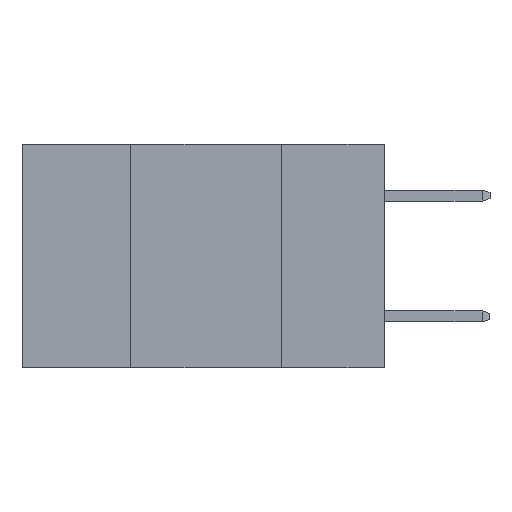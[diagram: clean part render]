
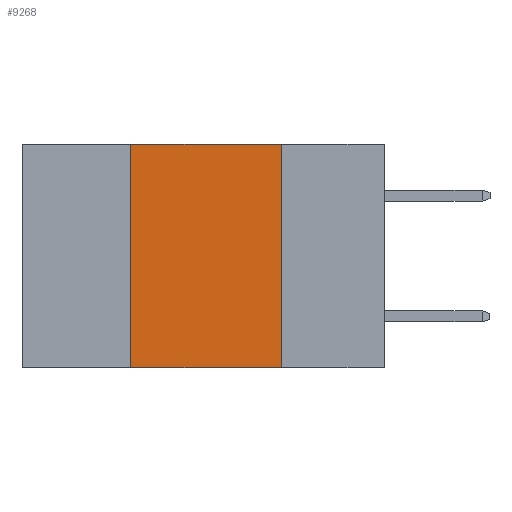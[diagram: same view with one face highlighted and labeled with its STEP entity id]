
A CAD part, left-side view. The second image highlights one B-rep face of the part: STEP entity #9268.
In plain terms, the highlighted planar face has unit normal (-1, 0, 0).
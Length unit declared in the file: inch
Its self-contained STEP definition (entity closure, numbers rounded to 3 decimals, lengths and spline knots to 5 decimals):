
#30 = EDGE_LOOP ( 'NONE', ( #9374, #10619, #9233, #5030 ) ) ;
#102 = VERTEX_POINT ( 'NONE', #7664 ) ;
#133 = CARTESIAN_POINT ( 'NONE',  ( 0., 0.42, 0. ) ) ;
#432 = CARTESIAN_POINT ( 'NONE',  ( 0., 0.6, -0.37 ) ) ;
#594 = CARTESIAN_POINT ( 'NONE',  ( 0., 0.42, 0. ) ) ;
#979 = EDGE_CURVE ( 'NONE', #102, #9115, #9741, .T. ) ;
#1003 = DIRECTION ( 'NONE',  ( 0., 0., 1. ) ) ;
#1593 = DIRECTION ( 'NONE',  ( 0., -1., 0. ) ) ;
#1744 = VECTOR ( 'NONE', #5534, 39.37008 ) ;
#2092 = AXIS2_PLACEMENT_3D ( 'NONE', #9020, #3743, #9863 ) ;
#2441 = LINE ( 'NONE', #133, #8982 ) ;
#2707 = VECTOR ( 'NONE', #3773, 39.37008 ) ;
#2812 = PLANE ( 'NONE',  #2092 ) ;
#3152 = VERTEX_POINT ( 'NONE', #594 ) ;
#3743 = DIRECTION ( 'NONE',  ( 1., 0., 0. ) ) ;
#3773 = DIRECTION ( 'NONE',  ( 0., -1., 0. ) ) ;
#3860 = LINE ( 'NONE', #4650, #1744 ) ;
#4650 = CARTESIAN_POINT ( 'NONE',  ( 0., 0.17, 0. ) ) ;
#5030 = ORIENTED_EDGE ( 'NONE', *, *, #979, .T. ) ;
#5378 = LINE ( 'NONE', #6963, #7765 ) ;
#5534 = DIRECTION ( 'NONE',  ( 0., 0., -1. ) ) ;
#5573 = CARTESIAN_POINT ( 'NONE',  ( 0., 0.17, 0. ) ) ;
#5905 = EDGE_CURVE ( 'NONE', #3152, #10644, #5378, .T. ) ;
#6963 = CARTESIAN_POINT ( 'NONE',  ( 0., 0.6, 0. ) ) ;
#7664 = CARTESIAN_POINT ( 'NONE',  ( 0., 0.42, -0.37 ) ) ;
#7765 = VECTOR ( 'NONE', #1593, 39.37008 ) ;
#8982 = VECTOR ( 'NONE', #1003, 39.37008 ) ;
#9020 = CARTESIAN_POINT ( 'NONE',  ( 0., 0.6, 0. ) ) ;
#9115 = VERTEX_POINT ( 'NONE', #10487 ) ;
#9233 = ORIENTED_EDGE ( 'NONE', *, *, #9871, .F. ) ;
#9268 = ADVANCED_FACE ( 'NONE', ( #10863 ), #2812, .F. ) ;
#9374 = ORIENTED_EDGE ( 'NONE', *, *, #10616, .F. ) ;
#9741 = LINE ( 'NONE', #432, #2707 ) ;
#9863 = DIRECTION ( 'NONE',  ( 0., 0., -1. ) ) ;
#9871 = EDGE_CURVE ( 'NONE', #102, #3152, #2441, .T. ) ;
#10487 = CARTESIAN_POINT ( 'NONE',  ( 0., 0.17, -0.37 ) ) ;
#10616 = EDGE_CURVE ( 'NONE', #10644, #9115, #3860, .T. ) ;
#10619 = ORIENTED_EDGE ( 'NONE', *, *, #5905, .F. ) ;
#10644 = VERTEX_POINT ( 'NONE', #5573 ) ;
#10863 = FACE_OUTER_BOUND ( 'NONE', #30, .T. ) ;
